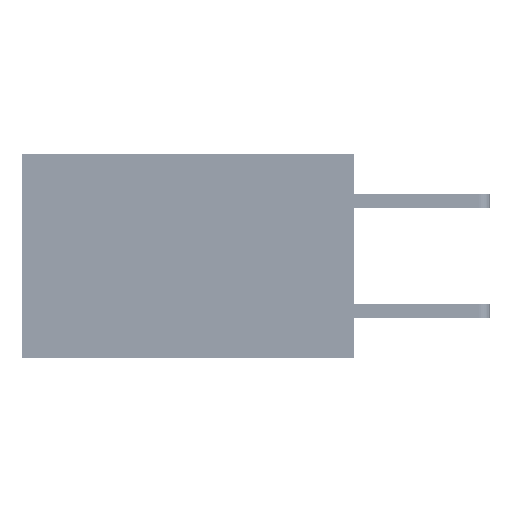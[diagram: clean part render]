
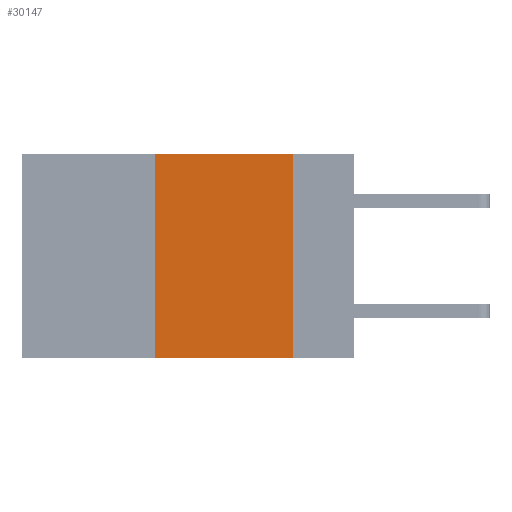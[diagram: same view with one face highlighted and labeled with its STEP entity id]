
A CAD part, left-side view. The second image highlights one B-rep face of the part: STEP entity #30147.
In plain terms, the highlighted planar face has unit normal (-1, 0, 0).
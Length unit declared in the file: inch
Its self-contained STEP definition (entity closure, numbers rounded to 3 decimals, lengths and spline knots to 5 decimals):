
#226 = EDGE_CURVE ( 'NONE', #29641, #11004, #24795, .T. ) ;
#608 = DIRECTION ( 'NONE',  ( 0., -1., 0. ) ) ;
#1185 = AXIS2_PLACEMENT_3D ( 'NONE', #5595, #28295, #34160 ) ;
#2730 = ORIENTED_EDGE ( 'NONE', *, *, #226, .F. ) ;
#3121 = EDGE_CURVE ( 'NONE', #24986, #31347, #8815, .T. ) ;
#5595 = CARTESIAN_POINT ( 'NONE',  ( 0., 0.6, 0. ) ) ;
#6008 = CARTESIAN_POINT ( 'NONE',  ( 0., 0.6, -0.37 ) ) ;
#6278 = VECTOR ( 'NONE', #608, 39.37008 ) ;
#6301 = EDGE_LOOP ( 'NONE', ( #29840, #2730, #7542, #7620 ) ) ;
#7542 = ORIENTED_EDGE ( 'NONE', *, *, #26496, .F. ) ;
#7620 = ORIENTED_EDGE ( 'NONE', *, *, #3121, .T. ) ;
#8815 = LINE ( 'NONE', #6008, #6278 ) ;
#10100 = CARTESIAN_POINT ( 'NONE',  ( 0., 0.11, -0.37 ) ) ;
#11004 = VERTEX_POINT ( 'NONE', #41100 ) ;
#14125 = DIRECTION ( 'NONE',  ( 0., 0., 1. ) ) ;
#16176 = VECTOR ( 'NONE', #27515, 39.37008 ) ;
#18427 = FACE_OUTER_BOUND ( 'NONE', #6301, .T. ) ;
#18467 = CARTESIAN_POINT ( 'NONE',  ( 0., 0.36, -0.37 ) ) ;
#20463 = LINE ( 'NONE', #24697, #26049 ) ;
#22943 = EDGE_CURVE ( 'NONE', #11004, #31347, #20463, .T. ) ;
#23544 = VECTOR ( 'NONE', #14125, 39.37008 ) ;
#24602 = LINE ( 'NONE', #40081, #23544 ) ;
#24697 = CARTESIAN_POINT ( 'NONE',  ( 0., 0.11, 0. ) ) ;
#24795 = LINE ( 'NONE', #28092, #16176 ) ;
#24986 = VERTEX_POINT ( 'NONE', #18467 ) ;
#26049 = VECTOR ( 'NONE', #41152, 39.37008 ) ;
#26496 = EDGE_CURVE ( 'NONE', #24986, #29641, #24602, .T. ) ;
#27515 = DIRECTION ( 'NONE',  ( 0., -1., 0. ) ) ;
#28092 = CARTESIAN_POINT ( 'NONE',  ( 0., 0.6, 0. ) ) ;
#28295 = DIRECTION ( 'NONE',  ( 1., 0., 0. ) ) ;
#29641 = VERTEX_POINT ( 'NONE', #29810 ) ;
#29810 = CARTESIAN_POINT ( 'NONE',  ( 0., 0.36, 0. ) ) ;
#29840 = ORIENTED_EDGE ( 'NONE', *, *, #22943, .F. ) ;
#30147 = ADVANCED_FACE ( 'NONE', ( #18427 ), #40920, .F. ) ;
#31347 = VERTEX_POINT ( 'NONE', #10100 ) ;
#34160 = DIRECTION ( 'NONE',  ( 0., 0., -1. ) ) ;
#40081 = CARTESIAN_POINT ( 'NONE',  ( 0., 0.36, 0. ) ) ;
#40920 = PLANE ( 'NONE',  #1185 ) ;
#41100 = CARTESIAN_POINT ( 'NONE',  ( 0., 0.11, 0. ) ) ;
#41152 = DIRECTION ( 'NONE',  ( 0., 0., -1. ) ) ;
